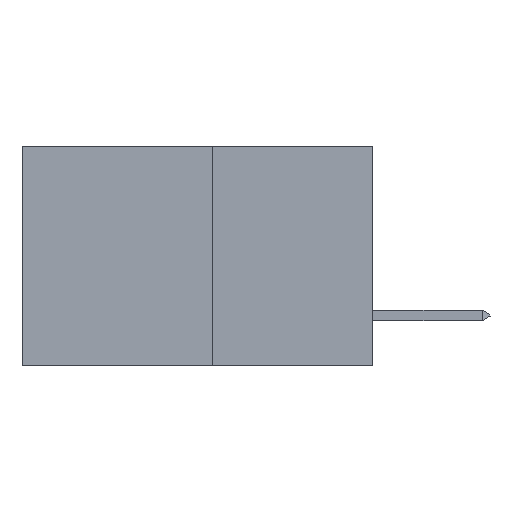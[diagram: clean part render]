
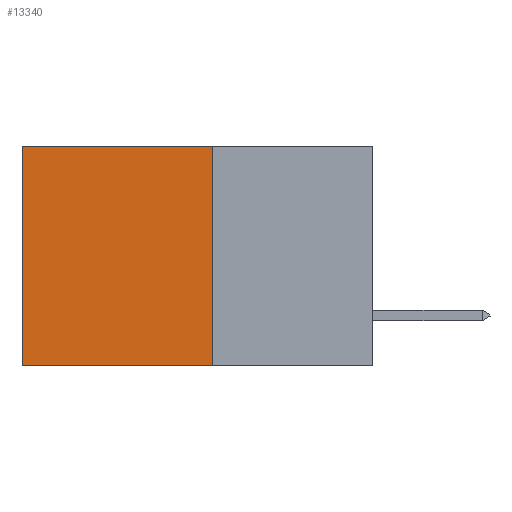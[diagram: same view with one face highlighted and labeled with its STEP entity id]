
A CAD part, left-side view. The second image highlights one B-rep face of the part: STEP entity #13340.
In plain terms, the highlighted planar face has unit normal (-1, 0, 0).
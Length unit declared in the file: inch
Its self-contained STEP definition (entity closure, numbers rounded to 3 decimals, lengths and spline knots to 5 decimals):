
#92 = EDGE_CURVE ( 'NONE', #11680, #954, #10258, .T. ) ;
#954 = VERTEX_POINT ( 'NONE', #14226 ) ;
#1995 = EDGE_CURVE ( 'NONE', #11680, #6994, #6546, .T. ) ;
#2469 = EDGE_CURVE ( 'NONE', #954, #11968, #14801, .T. ) ;
#2588 = EDGE_CURVE ( 'NONE', #6994, #11968, #5318, .T. ) ;
#3207 = VECTOR ( 'NONE', #14721, 39.37008 ) ;
#3999 = DIRECTION ( 'NONE',  ( 0., 0., -1. ) ) ;
#5318 = LINE ( 'NONE', #6741, #8266 ) ;
#5598 = CARTESIAN_POINT ( 'NONE',  ( 0.277, 0.59, 0. ) ) ;
#6546 = LINE ( 'NONE', #14918, #3207 ) ;
#6697 = DIRECTION ( 'NONE',  ( 0., 0., -1. ) ) ;
#6741 = CARTESIAN_POINT ( 'NONE',  ( 0.277, 0.59, -0.37 ) ) ;
#6994 = VERTEX_POINT ( 'NONE', #5598 ) ;
#7163 = ORIENTED_EDGE ( 'NONE', *, *, #2588, .T. ) ;
#7766 = ORIENTED_EDGE ( 'NONE', *, *, #92, .F. ) ;
#8261 = CARTESIAN_POINT ( 'NONE',  ( 0.277, 0.27, -0.37 ) ) ;
#8266 = VECTOR ( 'NONE', #6697, 39.37008 ) ;
#8374 = DIRECTION ( 'NONE',  ( 0., 0., -1. ) ) ;
#8404 = DIRECTION ( 'NONE',  ( 0., 1., 0. ) ) ;
#8570 = CARTESIAN_POINT ( 'NONE',  ( 0.277, 0.27, -0.37 ) ) ;
#9024 = AXIS2_PLACEMENT_3D ( 'NONE', #16510, #11524, #3999 ) ;
#10258 = LINE ( 'NONE', #8261, #16560 ) ;
#10707 = ORIENTED_EDGE ( 'NONE', *, *, #1995, .T. ) ;
#11248 = CARTESIAN_POINT ( 'NONE',  ( 0.277, 0.59, -0.37 ) ) ;
#11440 = VECTOR ( 'NONE', #8404, 39.37008 ) ;
#11524 = DIRECTION ( 'NONE',  ( 1., 0., 0. ) ) ;
#11680 = VERTEX_POINT ( 'NONE', #14582 ) ;
#11968 = VERTEX_POINT ( 'NONE', #11248 ) ;
#13340 = ADVANCED_FACE ( 'NONE', ( #13444 ), #15267, .F. ) ;
#13424 = EDGE_LOOP ( 'NONE', ( #7163, #15763, #7766, #10707 ) ) ;
#13444 = FACE_OUTER_BOUND ( 'NONE', #13424, .T. ) ;
#14226 = CARTESIAN_POINT ( 'NONE',  ( 0.277, 0.27, -0.37 ) ) ;
#14582 = CARTESIAN_POINT ( 'NONE',  ( 0.277, 0.27, 0. ) ) ;
#14721 = DIRECTION ( 'NONE',  ( 0., 1., 0. ) ) ;
#14801 = LINE ( 'NONE', #8570, #11440 ) ;
#14918 = CARTESIAN_POINT ( 'NONE',  ( 0.277, 0.27, 0. ) ) ;
#15267 = PLANE ( 'NONE',  #9024 ) ;
#15763 = ORIENTED_EDGE ( 'NONE', *, *, #2469, .F. ) ;
#16510 = CARTESIAN_POINT ( 'NONE',  ( 0.277, 0.27, -0.37 ) ) ;
#16560 = VECTOR ( 'NONE', #8374, 39.37008 ) ;
